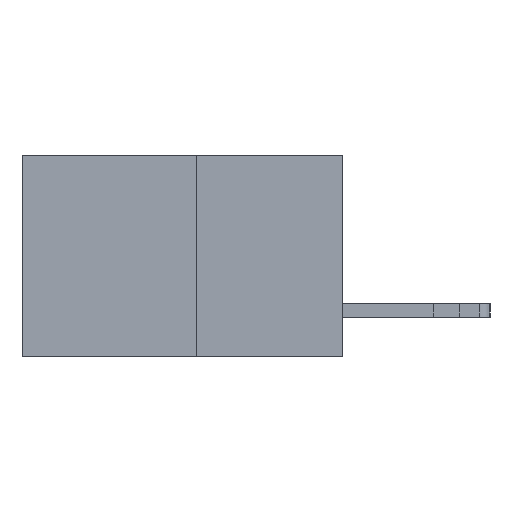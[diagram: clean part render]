
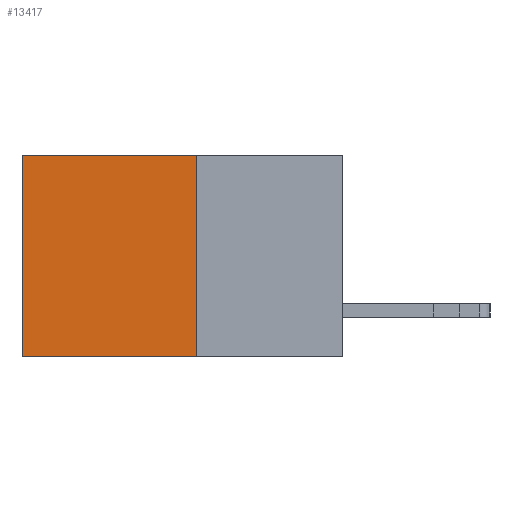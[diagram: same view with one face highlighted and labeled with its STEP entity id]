
A CAD part, left-side view. The second image highlights one B-rep face of the part: STEP entity #13417.
In plain terms, the highlighted planar face has unit normal (-1, 0, 0).
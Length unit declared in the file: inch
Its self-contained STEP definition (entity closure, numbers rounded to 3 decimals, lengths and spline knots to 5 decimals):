
#860 = AXIS2_PLACEMENT_3D ( 'NONE', #11591, #12874, #5164 ) ;
#992 = EDGE_CURVE ( 'NONE', #1260, #12467, #14700, .T. ) ;
#1260 = VERTEX_POINT ( 'NONE', #5620 ) ;
#1500 = CARTESIAN_POINT ( 'NONE',  ( 0.277, 0.59, -0.37 ) ) ;
#1602 = FACE_OUTER_BOUND ( 'NONE', #2912, .T. ) ;
#2255 = ORIENTED_EDGE ( 'NONE', *, *, #2471, .F. ) ;
#2400 = CARTESIAN_POINT ( 'NONE',  ( 0.277, 0.27, -0.37 ) ) ;
#2471 = EDGE_CURVE ( 'NONE', #6680, #3116, #14657, .T. ) ;
#2912 = EDGE_LOOP ( 'NONE', ( #4827, #4895, #2255, #4256 ) ) ;
#2920 = LINE ( 'NONE', #2400, #6053 ) ;
#3116 = VERTEX_POINT ( 'NONE', #11229 ) ;
#4256 = ORIENTED_EDGE ( 'NONE', *, *, #13885, .T. ) ;
#4378 = VECTOR ( 'NONE', #5735, 39.37008 ) ;
#4827 = ORIENTED_EDGE ( 'NONE', *, *, #992, .T. ) ;
#4895 = ORIENTED_EDGE ( 'NONE', *, *, #14155, .F. ) ;
#5164 = DIRECTION ( 'NONE',  ( 0., 0., -1. ) ) ;
#5620 = CARTESIAN_POINT ( 'NONE',  ( 0.277, 0.59, 0. ) ) ;
#5735 = DIRECTION ( 'NONE',  ( 0., 0., -1. ) ) ;
#6053 = VECTOR ( 'NONE', #6401, 39.37008 ) ;
#6401 = DIRECTION ( 'NONE',  ( 0., 1., 0. ) ) ;
#6680 = VERTEX_POINT ( 'NONE', #9638 ) ;
#7437 = LINE ( 'NONE', #14576, #13872 ) ;
#9015 = PLANE ( 'NONE',  #860 ) ;
#9638 = CARTESIAN_POINT ( 'NONE',  ( 0.277, 0.27, 0. ) ) ;
#10677 = DIRECTION ( 'NONE',  ( 0., 0., -1. ) ) ;
#11229 = CARTESIAN_POINT ( 'NONE',  ( 0.277, 0.27, -0.37 ) ) ;
#11591 = CARTESIAN_POINT ( 'NONE',  ( 0.277, 0.27, -0.37 ) ) ;
#11736 = VECTOR ( 'NONE', #10677, 39.37008 ) ;
#12250 = CARTESIAN_POINT ( 'NONE',  ( 0.277, 0.27, -0.37 ) ) ;
#12467 = VERTEX_POINT ( 'NONE', #1500 ) ;
#12874 = DIRECTION ( 'NONE',  ( 1., 0., 0. ) ) ;
#13417 = ADVANCED_FACE ( 'NONE', ( #1602 ), #9015, .F. ) ;
#13872 = VECTOR ( 'NONE', #15802, 39.37008 ) ;
#13885 = EDGE_CURVE ( 'NONE', #6680, #1260, #7437, .T. ) ;
#14155 = EDGE_CURVE ( 'NONE', #3116, #12467, #2920, .T. ) ;
#14576 = CARTESIAN_POINT ( 'NONE',  ( 0.277, 0.27, 0. ) ) ;
#14657 = LINE ( 'NONE', #12250, #4378 ) ;
#14700 = LINE ( 'NONE', #16884, #11736 ) ;
#15802 = DIRECTION ( 'NONE',  ( 0., 1., 0. ) ) ;
#16884 = CARTESIAN_POINT ( 'NONE',  ( 0.277, 0.59, -0.37 ) ) ;
